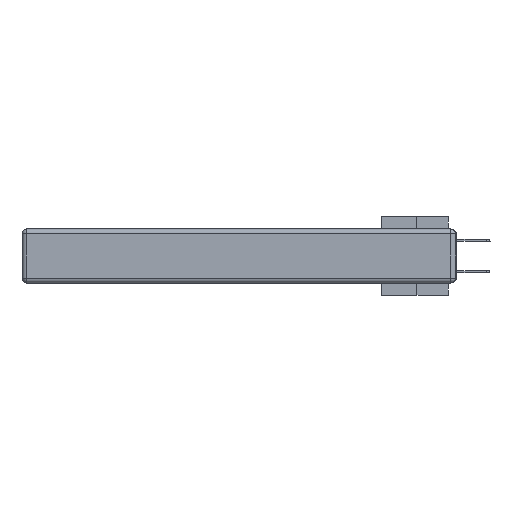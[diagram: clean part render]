
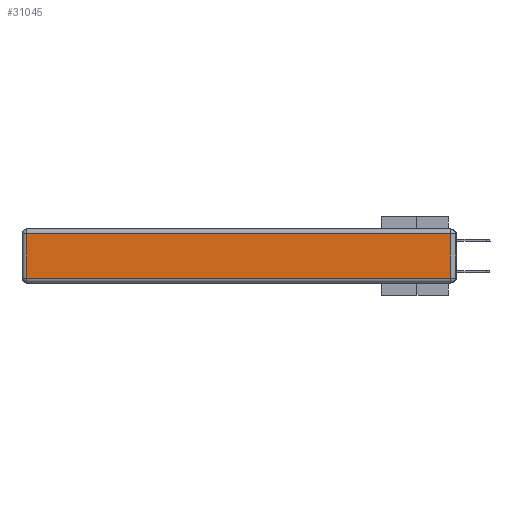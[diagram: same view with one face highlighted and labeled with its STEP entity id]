
A CAD part, left-side view. The second image highlights one B-rep face of the part: STEP entity #31045.
In plain terms, the highlighted planar face has unit normal (-1, 0, 0).
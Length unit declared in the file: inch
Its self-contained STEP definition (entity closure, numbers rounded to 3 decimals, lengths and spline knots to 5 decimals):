
#659 = VECTOR ( 'NONE', #33424, 39.37008 ) ;
#2723 = VECTOR ( 'NONE', #5148, 39.37008 ) ;
#3229 = VERTEX_POINT ( 'NONE', #18965 ) ;
#3236 = LINE ( 'NONE', #11119, #18769 ) ;
#3869 = DIRECTION ( 'NONE',  ( 0., 1., 0. ) ) ;
#4097 = CARTESIAN_POINT ( 'NONE',  ( 0., 2.75, -0.03 ) ) ;
#4113 = EDGE_CURVE ( 'NONE', #3229, #27480, #7983, .T. ) ;
#4732 = FACE_OUTER_BOUND ( 'NONE', #14752, .T. ) ;
#5148 = DIRECTION ( 'NONE',  ( 0., 0., -1. ) ) ;
#6628 = CARTESIAN_POINT ( 'NONE',  ( 0., 2.72, -0.03 ) ) ;
#7983 = LINE ( 'NONE', #12498, #659 ) ;
#8493 = CARTESIAN_POINT ( 'NONE',  ( 0., 0., -0.343 ) ) ;
#9932 = ORIENTED_EDGE ( 'NONE', *, *, #4113, .T. ) ;
#11057 = EDGE_CURVE ( 'NONE', #27480, #21579, #3236, .T. ) ;
#11119 = CARTESIAN_POINT ( 'NONE',  ( 0., 0.03, -0.343 ) ) ;
#12498 = CARTESIAN_POINT ( 'NONE',  ( 0., 0., -0.313 ) ) ;
#13690 = VECTOR ( 'NONE', #3869, 39.37008 ) ;
#14752 = EDGE_LOOP ( 'NONE', ( #9932, #23458, #32515, #31348 ) ) ;
#16419 = DIRECTION ( 'NONE',  ( 0., 0., 1. ) ) ;
#17845 = VERTEX_POINT ( 'NONE', #6628 ) ;
#18642 = LINE ( 'NONE', #30924, #2723 ) ;
#18769 = VECTOR ( 'NONE', #24115, 39.37008 ) ;
#18965 = CARTESIAN_POINT ( 'NONE',  ( 0., 2.72, -0.313 ) ) ;
#20710 = LINE ( 'NONE', #4097, #13690 ) ;
#21579 = VERTEX_POINT ( 'NONE', #32081 ) ;
#22046 = DIRECTION ( 'NONE',  ( -1., 0., 0. ) ) ;
#22301 = EDGE_CURVE ( 'NONE', #21579, #17845, #20710, .T. ) ;
#23458 = ORIENTED_EDGE ( 'NONE', *, *, #11057, .T. ) ;
#24115 = DIRECTION ( 'NONE',  ( 0., 0., 1. ) ) ;
#27157 = EDGE_CURVE ( 'NONE', #17845, #3229, #18642, .T. ) ;
#27480 = VERTEX_POINT ( 'NONE', #32415 ) ;
#28403 = AXIS2_PLACEMENT_3D ( 'NONE', #8493, #22046, #16419 ) ;
#30924 = CARTESIAN_POINT ( 'NONE',  ( 0., 2.72, -0.343 ) ) ;
#31045 = ADVANCED_FACE ( 'NONE', ( #4732 ), #32484, .T. ) ;
#31348 = ORIENTED_EDGE ( 'NONE', *, *, #27157, .T. ) ;
#32081 = CARTESIAN_POINT ( 'NONE',  ( 0., 0.03, -0.03 ) ) ;
#32415 = CARTESIAN_POINT ( 'NONE',  ( 0., 0.03, -0.313 ) ) ;
#32484 = PLANE ( 'NONE',  #28403 ) ;
#32515 = ORIENTED_EDGE ( 'NONE', *, *, #22301, .T. ) ;
#33424 = DIRECTION ( 'NONE',  ( 0., -1., 0. ) ) ;
